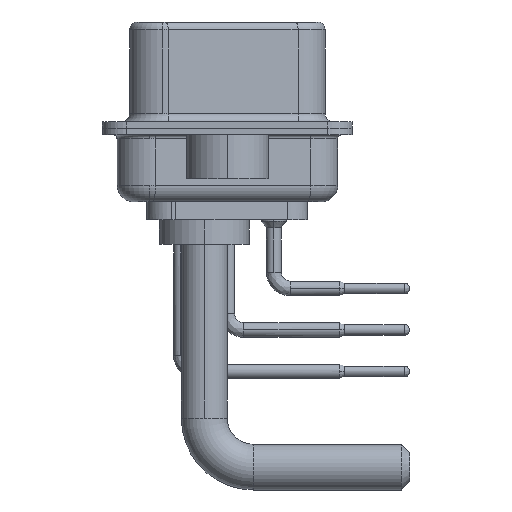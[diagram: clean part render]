
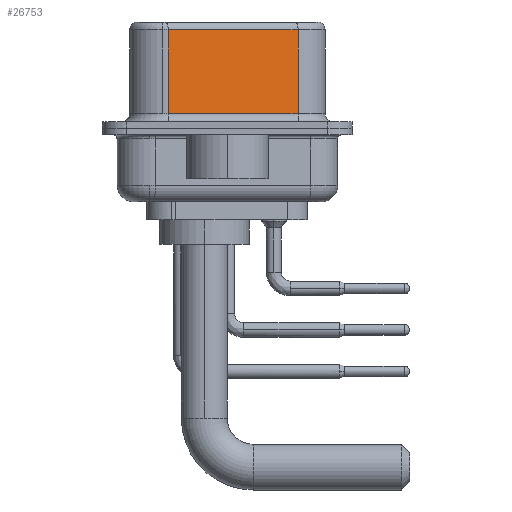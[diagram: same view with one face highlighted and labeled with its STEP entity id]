
A CAD part, left-side view. The second image highlights one B-rep face of the part: STEP entity #26753.
In plain terms, the highlighted planar face has unit normal (-0.985, -0.174, 0).
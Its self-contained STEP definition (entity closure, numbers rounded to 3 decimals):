
#164 = DIRECTION ( 'NONE',  ( -0.174, 0.985, 0. ) ) ;
#1295 = CARTESIAN_POINT ( 'NONE',  ( 5.132, -4.322, 0.9 ) ) ;
#1793 = VECTOR ( 'NONE', #3456, 1000. ) ;
#2627 = LINE ( 'NONE', #12676, #2766 ) ;
#2766 = VECTOR ( 'NONE', #10094, 1000. ) ;
#3456 = DIRECTION ( 'NONE',  ( -0.174, 0.985, 0. ) ) ;
#5531 = CARTESIAN_POINT ( 'NONE',  ( 5.132, -4.322, 6.52 ) ) ;
#6403 = LINE ( 'NONE', #24752, #1793 ) ;
#6481 = CARTESIAN_POINT ( 'NONE',  ( 3.73, 3.628, 6.52 ) ) ;
#8325 = VERTEX_POINT ( 'NONE', #1295 ) ;
#9846 = CARTESIAN_POINT ( 'NONE',  ( 3.73, 3.628, 6.02 ) ) ;
#10094 = DIRECTION ( 'NONE',  ( 0.174, -0.985, 0. ) ) ;
#12281 = ORIENTED_EDGE ( 'NONE', *, *, #25741, .T. ) ;
#12582 = ORIENTED_EDGE ( 'NONE', *, *, #13984, .T. ) ;
#12676 = CARTESIAN_POINT ( 'NONE',  ( 5.132, -4.322, 0.9 ) ) ;
#13089 = EDGE_CURVE ( 'NONE', #29591, #18674, #14625, .T. ) ;
#13638 = CARTESIAN_POINT ( 'NONE',  ( 5.132, -4.322, 6.52 ) ) ;
#13984 = EDGE_CURVE ( 'NONE', #24886, #29591, #6403, .T. ) ;
#14608 = ORIENTED_EDGE ( 'NONE', *, *, #27577, .F. ) ;
#14625 = LINE ( 'NONE', #6481, #32160 ) ;
#14992 = VECTOR ( 'NONE', #29892, 1000. ) ;
#15944 = PLANE ( 'NONE',  #23769 ) ;
#15977 = ORIENTED_EDGE ( 'NONE', *, *, #13089, .T. ) ;
#18674 = VERTEX_POINT ( 'NONE', #33440 ) ;
#18698 = DIRECTION ( 'NONE',  ( 0.985, 0.174, 0. ) ) ;
#18996 = LINE ( 'NONE', #13638, #14992 ) ;
#20540 = CARTESIAN_POINT ( 'NONE',  ( 5.132, -4.322, 6.02 ) ) ;
#23769 = AXIS2_PLACEMENT_3D ( 'NONE', #5531, #18698, #164 ) ;
#23883 = FACE_OUTER_BOUND ( 'NONE', #32453, .T. ) ;
#24752 = CARTESIAN_POINT ( 'NONE',  ( 5.132, -4.322, 6.02 ) ) ;
#24886 = VERTEX_POINT ( 'NONE', #20540 ) ;
#25162 = DIRECTION ( 'NONE',  ( 0., 0., -1. ) ) ;
#25741 = EDGE_CURVE ( 'NONE', #18674, #8325, #2627, .T. ) ;
#26753 = ADVANCED_FACE ( 'NONE', ( #23883 ), #15944, .F. ) ;
#27577 = EDGE_CURVE ( 'NONE', #24886, #8325, #18996, .T. ) ;
#29591 = VERTEX_POINT ( 'NONE', #9846 ) ;
#29892 = DIRECTION ( 'NONE',  ( 0., 0., -1. ) ) ;
#32160 = VECTOR ( 'NONE', #25162, 1000. ) ;
#32453 = EDGE_LOOP ( 'NONE', ( #14608, #12582, #15977, #12281 ) ) ;
#33440 = CARTESIAN_POINT ( 'NONE',  ( 3.73, 3.628, 0.9 ) ) ;
